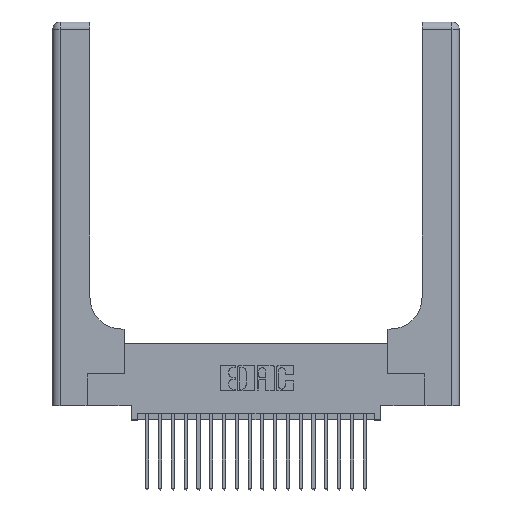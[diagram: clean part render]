
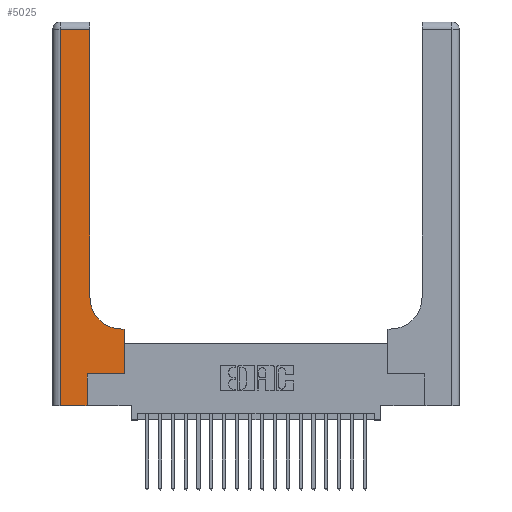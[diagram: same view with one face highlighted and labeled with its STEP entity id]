
A CAD part, top view. The second image highlights one B-rep face of the part: STEP entity #5025.
In plain terms, the highlighted planar face has unit normal (0, 0, 1).
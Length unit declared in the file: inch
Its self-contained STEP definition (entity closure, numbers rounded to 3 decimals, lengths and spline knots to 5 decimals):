
#267 = VERTEX_POINT ( 'NONE', #17729 ) ;
#723 = VERTEX_POINT ( 'NONE', #19038 ) ;
#774 = DIRECTION ( 'NONE',  ( -1., 0., 0. ) ) ;
#1062 = CARTESIAN_POINT ( 'NONE',  ( 0.06, 2.94, 0.37 ) ) ;
#1623 = CARTESIAN_POINT ( 'NONE',  ( 0.2915, 2.94, 0.37 ) ) ;
#1830 = LINE ( 'NONE', #14590, #19316 ) ;
#1959 = VECTOR ( 'NONE', #9916, 39.37008 ) ;
#2017 = DIRECTION ( 'NONE',  ( 0., 1., 0. ) ) ;
#2214 = VERTEX_POINT ( 'NONE', #1623 ) ;
#3760 = DIRECTION ( 'NONE',  ( 0., 0., -1. ) ) ;
#3853 = EDGE_LOOP ( 'NONE', ( #19527, #15872, #7273, #12105, #20158, #5415, #21367, #8282, #9839 ) ) ;
#4142 = CARTESIAN_POINT ( 'NONE',  ( 0.2915, 3., 0.37 ) ) ;
#4809 = LINE ( 'NONE', #4142, #8880 ) ;
#4839 = CARTESIAN_POINT ( 'NONE',  ( 0.06, 3., 0.37 ) ) ;
#5025 = ADVANCED_FACE ( 'NONE', ( #13246 ), #7893, .F. ) ;
#5029 = EDGE_CURVE ( 'NONE', #19622, #19924, #8611, .T. ) ;
#5415 = ORIENTED_EDGE ( 'NONE', *, *, #11644, .T. ) ;
#5717 = EDGE_CURVE ( 'NONE', #13004, #7687, #19137, .T. ) ;
#5899 = DIRECTION ( 'NONE',  ( 0., 1., 0. ) ) ;
#7273 = ORIENTED_EDGE ( 'NONE', *, *, #10554, .T. ) ;
#7687 = VERTEX_POINT ( 'NONE', #16207 ) ;
#7893 = PLANE ( 'NONE',  #9367 ) ;
#8282 = ORIENTED_EDGE ( 'NONE', *, *, #5029, .T. ) ;
#8296 = CIRCLE ( 'NONE', #21874, 0.25 ) ;
#8592 = LINE ( 'NONE', #4839, #12690 ) ;
#8611 = LINE ( 'NONE', #13148, #12708 ) ;
#8814 = LINE ( 'NONE', #13145, #20184 ) ;
#8880 = VECTOR ( 'NONE', #5899, 39.37008 ) ;
#9023 = EDGE_CURVE ( 'NONE', #7687, #20210, #10856, .T. ) ;
#9367 = AXIS2_PLACEMENT_3D ( 'NONE', #19984, #21739, #11391 ) ;
#9388 = VECTOR ( 'NONE', #17194, 39.37008 ) ;
#9839 = ORIENTED_EDGE ( 'NONE', *, *, #21220, .T. ) ;
#9916 = DIRECTION ( 'NONE',  ( 0., 1., 0. ) ) ;
#10265 = EDGE_CURVE ( 'NONE', #723, #2214, #4809, .T. ) ;
#10318 = VECTOR ( 'NONE', #2017, 39.37008 ) ;
#10517 = CARTESIAN_POINT ( 'NONE',  ( 0.5585, 0.25, 0.37 ) ) ;
#10554 = EDGE_CURVE ( 'NONE', #19543, #13004, #8592, .T. ) ;
#10830 = CARTESIAN_POINT ( 'NONE',  ( 0.269, 0., 0.37 ) ) ;
#10856 = LINE ( 'NONE', #10830, #10318 ) ;
#11354 = LINE ( 'NONE', #10517, #1959 ) ;
#11391 = DIRECTION ( 'NONE',  ( -1., 0., 0. ) ) ;
#11644 = EDGE_CURVE ( 'NONE', #20210, #267, #8814, .T. ) ;
#11806 = CARTESIAN_POINT ( 'NONE',  ( 0.06, 0., 0.37 ) ) ;
#12105 = ORIENTED_EDGE ( 'NONE', *, *, #5717, .T. ) ;
#12650 = CARTESIAN_POINT ( 'NONE',  ( 0.5415, 0.6, 0.37 ) ) ;
#12690 = VECTOR ( 'NONE', #22085, 39.37008 ) ;
#12708 = VECTOR ( 'NONE', #774, 39.37008 ) ;
#12719 = EDGE_CURVE ( 'NONE', #2214, #19543, #1830, .T. ) ;
#13004 = VERTEX_POINT ( 'NONE', #11806 ) ;
#13145 = CARTESIAN_POINT ( 'NONE',  ( 0.269, 0.25, 0.37 ) ) ;
#13148 = CARTESIAN_POINT ( 'NONE',  ( 0.2915, 0.6, 0.37 ) ) ;
#13246 = FACE_OUTER_BOUND ( 'NONE', #3853, .T. ) ;
#14189 = CARTESIAN_POINT ( 'NONE',  ( 0.5415, 0.85, 0.37 ) ) ;
#14590 = CARTESIAN_POINT ( 'NONE',  ( 0., 2.94, 0.37 ) ) ;
#15872 = ORIENTED_EDGE ( 'NONE', *, *, #12719, .T. ) ;
#15928 = DIRECTION ( 'NONE',  ( 1., 0., 0. ) ) ;
#16207 = CARTESIAN_POINT ( 'NONE',  ( 0.269, 0., 0.37 ) ) ;
#17194 = DIRECTION ( 'NONE',  ( 1., 0., 0. ) ) ;
#17618 = EDGE_CURVE ( 'NONE', #267, #19622, #11354, .T. ) ;
#17729 = CARTESIAN_POINT ( 'NONE',  ( 0.5585, 0.25, 0.37 ) ) ;
#19038 = CARTESIAN_POINT ( 'NONE',  ( 0.2915, 0.85, 0.37 ) ) ;
#19137 = LINE ( 'NONE', #20665, #9388 ) ;
#19316 = VECTOR ( 'NONE', #21455, 39.37008 ) ;
#19527 = ORIENTED_EDGE ( 'NONE', *, *, #10265, .T. ) ;
#19543 = VERTEX_POINT ( 'NONE', #1062 ) ;
#19622 = VERTEX_POINT ( 'NONE', #22142 ) ;
#19924 = VERTEX_POINT ( 'NONE', #12650 ) ;
#19984 = CARTESIAN_POINT ( 'NONE',  ( 0., 3., 0.37 ) ) ;
#20158 = ORIENTED_EDGE ( 'NONE', *, *, #9023, .T. ) ;
#20184 = VECTOR ( 'NONE', #21738, 39.37008 ) ;
#20210 = VERTEX_POINT ( 'NONE', #21977 ) ;
#20665 = CARTESIAN_POINT ( 'NONE',  ( 0., 0., 0.37 ) ) ;
#21220 = EDGE_CURVE ( 'NONE', #19924, #723, #8296, .T. ) ;
#21367 = ORIENTED_EDGE ( 'NONE', *, *, #17618, .T. ) ;
#21455 = DIRECTION ( 'NONE',  ( -1., 0., 0. ) ) ;
#21738 = DIRECTION ( 'NONE',  ( 1., 0., 0. ) ) ;
#21739 = DIRECTION ( 'NONE',  ( 0., 0., -1. ) ) ;
#21874 = AXIS2_PLACEMENT_3D ( 'NONE', #14189, #3760, #15928 ) ;
#21977 = CARTESIAN_POINT ( 'NONE',  ( 0.269, 0.25, 0.37 ) ) ;
#22085 = DIRECTION ( 'NONE',  ( 0., -1., 0. ) ) ;
#22142 = CARTESIAN_POINT ( 'NONE',  ( 0.5585, 0.6, 0.37 ) ) ;
